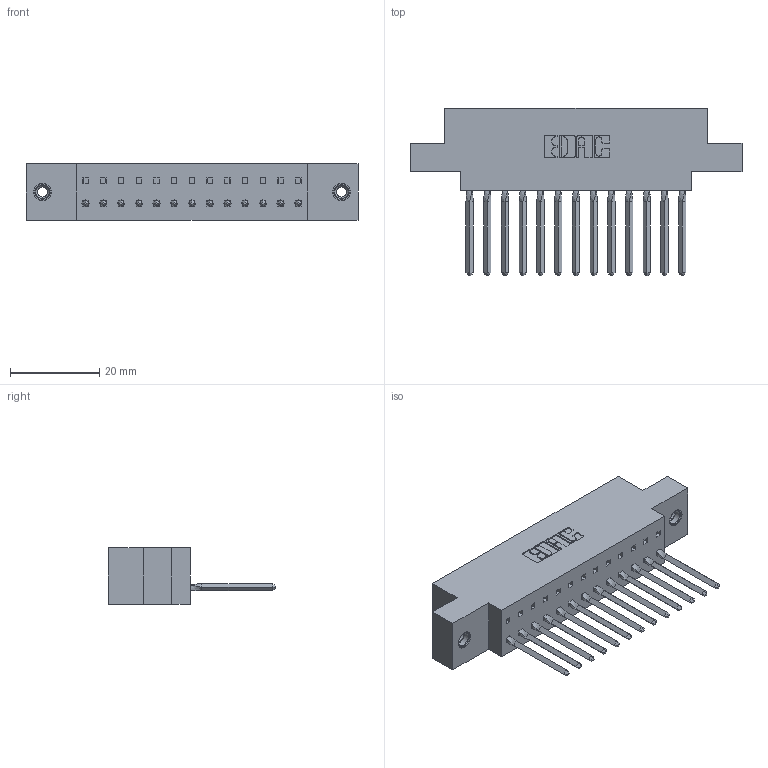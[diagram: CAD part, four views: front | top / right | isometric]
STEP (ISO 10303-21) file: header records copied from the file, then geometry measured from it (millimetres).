
FILE_DESCRIPTION (( 'STEP AP203' ), '1' );
FILE_NAME ('317-013-541-678.STEP', '2020-02-27T14:28:44', ( '' ), ( '' ), 'SwSTEP 2.0', 'SolidWorks 2016', '' );
FILE_SCHEMA (( 'CONFIG_CONTROL_DESIGN' ));
Length unit declared in the file: inch
Products named in the file (4): 317-290-002_541; 345-250-001_345-250-003-102; 317-013-541-678; 317 Part_.156 Dia - TI
Assembly tree (16 placements, depth 2):
  317-013-541-678
    317 Part_.156 Dia - TI
    317-290-002_541  x13
    345-250-001_345-250-003-102  x2
Bounding box: 74.22 x 37.34 x 12.7 mm (x, y, z)
Volume: 11137.6 mm3; surface area: 14792.8 mm2
Topology: 16 solids, 16 shells, 2138 faces, 6053 edges, 3932 vertices
Faces by surface type: plane 1702, cylinder 368, bspline 52, cone 12, torus 4
Entity records: 25155 total; most frequent: CARTESIAN_POINT 5067, ORIENTED_EDGE 4326, DIRECTION 3575, EDGE_CURVE 2163, LINE 1779, VECTOR 1779, VERTEX_POINT 1430, AXIS2_PLACEMENT_3D 898
